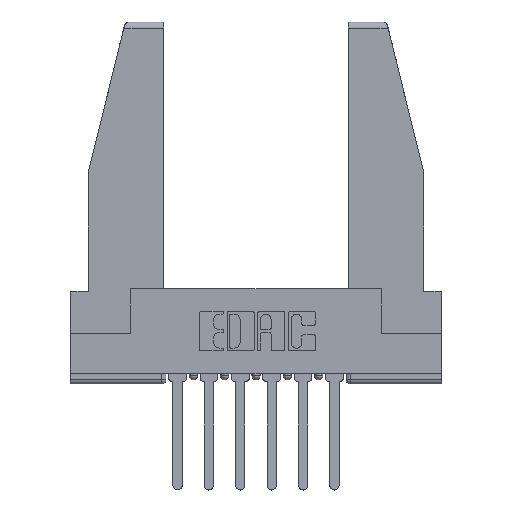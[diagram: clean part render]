
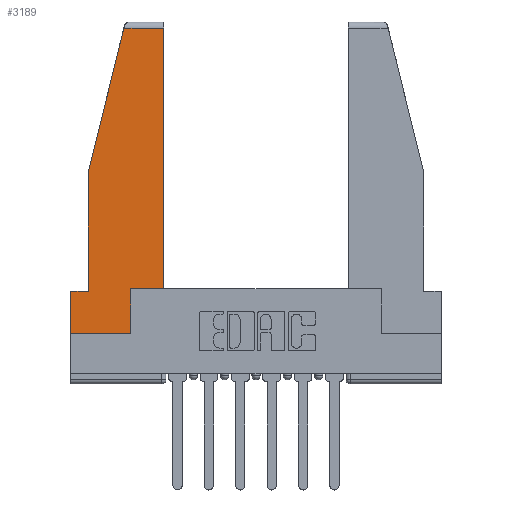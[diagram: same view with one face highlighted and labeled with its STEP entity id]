
A CAD part, top view. The second image highlights one B-rep face of the part: STEP entity #3189.
In plain terms, the highlighted planar face has unit normal (0, 0, 1).
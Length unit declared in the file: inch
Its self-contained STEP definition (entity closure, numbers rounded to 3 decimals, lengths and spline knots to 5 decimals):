
#70 = VERTEX_POINT ( 'NONE', #4856 ) ;
#126 = ORIENTED_EDGE ( 'NONE', *, *, #10428, .T. ) ;
#767 = VERTEX_POINT ( 'NONE', #4243 ) ;
#822 = EDGE_CURVE ( 'NONE', #12148, #7569, #9503, .T. ) ;
#844 = ORIENTED_EDGE ( 'NONE', *, *, #822, .T. ) ;
#858 = CARTESIAN_POINT ( 'NONE',  ( 0.086, 0.8, 0. ) ) ;
#1136 = PLANE ( 'NONE',  #5788 ) ;
#1160 = CARTESIAN_POINT ( 'NONE',  ( 0., 0., 0. ) ) ;
#1608 = CARTESIAN_POINT ( 'NONE',  ( 0., 0.21, 0. ) ) ;
#1762 = DIRECTION ( 'NONE',  ( 0., 1., 0. ) ) ;
#2064 = ORIENTED_EDGE ( 'NONE', *, *, #4403, .T. ) ;
#2156 = CARTESIAN_POINT ( 'NONE',  ( 0.271, 1.55, 0. ) ) ;
#2449 = DIRECTION ( 'NONE',  ( 1., 0., 0. ) ) ;
#3082 = DIRECTION ( 'NONE',  ( -0.239, -0.971, 0. ) ) ;
#3189 = ADVANCED_FACE ( 'NONE', ( #3199 ), #1136, .T. ) ;
#3199 = FACE_OUTER_BOUND ( 'NONE', #6763, .T. ) ;
#3532 = VECTOR ( 'NONE', #5253, 39.37008 ) ;
#3909 = EDGE_CURVE ( 'NONE', #70, #11465, #10698, .T. ) ;
#3946 = VECTOR ( 'NONE', #10074, 39.37008 ) ;
#4074 = EDGE_CURVE ( 'NONE', #6511, #70, #4246, .T. ) ;
#4205 = ORIENTED_EDGE ( 'NONE', *, *, #6234, .T. ) ;
#4243 = CARTESIAN_POINT ( 'NONE',  ( 0.297, 0., 0. ) ) ;
#4246 = LINE ( 'NONE', #8084, #3946 ) ;
#4403 = EDGE_CURVE ( 'NONE', #767, #12148, #9947, .T. ) ;
#4578 = CARTESIAN_POINT ( 'NONE',  ( 0.086, 0.21, 0. ) ) ;
#4725 = VECTOR ( 'NONE', #6793, 39.37008 ) ;
#4856 = CARTESIAN_POINT ( 'NONE',  ( 0.2636, 1.52, 0. ) ) ;
#5094 = CARTESIAN_POINT ( 'NONE',  ( 0., 0.21, 0. ) ) ;
#5253 = DIRECTION ( 'NONE',  ( 0., -1., 0. ) ) ;
#5254 = ORIENTED_EDGE ( 'NONE', *, *, #4074, .T. ) ;
#5375 = VECTOR ( 'NONE', #10734, 39.37008 ) ;
#5491 = CARTESIAN_POINT ( 'NONE',  ( 0.461, 0.223, 0. ) ) ;
#5518 = ORIENTED_EDGE ( 'NONE', *, *, #3909, .T. ) ;
#5684 = CARTESIAN_POINT ( 'NONE',  ( 0., 0.21, 0. ) ) ;
#5788 = AXIS2_PLACEMENT_3D ( 'NONE', #10563, #8725, #6898 ) ;
#5838 = VERTEX_POINT ( 'NONE', #8329 ) ;
#6207 = DIRECTION ( 'NONE',  ( 0., -1., 0. ) ) ;
#6234 = EDGE_CURVE ( 'NONE', #11465, #10917, #9386, .T. ) ;
#6461 = LINE ( 'NONE', #5094, #3532 ) ;
#6511 = VERTEX_POINT ( 'NONE', #9478 ) ;
#6543 = ORIENTED_EDGE ( 'NONE', *, *, #8089, .T. ) ;
#6763 = EDGE_LOOP ( 'NONE', ( #11177, #5254, #5518, #4205, #6543, #126, #9955, #2064, #844 ) ) ;
#6793 = DIRECTION ( 'NONE',  ( 1., 0., 0. ) ) ;
#6805 = LINE ( 'NONE', #5491, #7955 ) ;
#6880 = VECTOR ( 'NONE', #6207, 39.37008 ) ;
#6898 = DIRECTION ( 'NONE',  ( 1., 0., 0. ) ) ;
#6947 = CARTESIAN_POINT ( 'NONE',  ( 0.297, 0., 0. ) ) ;
#7335 = DIRECTION ( 'NONE',  ( -1., 0., 0. ) ) ;
#7569 = VERTEX_POINT ( 'NONE', #10974 ) ;
#7955 = VECTOR ( 'NONE', #1762, 39.37008 ) ;
#8084 = CARTESIAN_POINT ( 'NONE',  ( 0., 1.52, 0. ) ) ;
#8089 = EDGE_CURVE ( 'NONE', #10917, #9520, #11948, .T. ) ;
#8254 = VECTOR ( 'NONE', #7335, 39.37008 ) ;
#8329 = CARTESIAN_POINT ( 'NONE',  ( 0., 0., 0. ) ) ;
#8347 = CARTESIAN_POINT ( 'NONE',  ( 0.297, 0.223, 0. ) ) ;
#8725 = DIRECTION ( 'NONE',  ( 0., 0., 1. ) ) ;
#8764 = EDGE_CURVE ( 'NONE', #7569, #6511, #6805, .T. ) ;
#8935 = CARTESIAN_POINT ( 'NONE',  ( 0.086, 0.8, 0. ) ) ;
#9374 = VECTOR ( 'NONE', #3082, 39.37008 ) ;
#9386 = LINE ( 'NONE', #8935, #6880 ) ;
#9478 = CARTESIAN_POINT ( 'NONE',  ( 0.461, 1.52, 0. ) ) ;
#9503 = LINE ( 'NONE', #10431, #10085 ) ;
#9520 = VERTEX_POINT ( 'NONE', #5684 ) ;
#9707 = LINE ( 'NONE', #1160, #4725 ) ;
#9947 = LINE ( 'NONE', #6947, #5375 ) ;
#9955 = ORIENTED_EDGE ( 'NONE', *, *, #10263, .T. ) ;
#10074 = DIRECTION ( 'NONE',  ( -1., 0., 0. ) ) ;
#10085 = VECTOR ( 'NONE', #2449, 39.37008 ) ;
#10263 = EDGE_CURVE ( 'NONE', #5838, #767, #9707, .T. ) ;
#10428 = EDGE_CURVE ( 'NONE', #9520, #5838, #6461, .T. ) ;
#10431 = CARTESIAN_POINT ( 'NONE',  ( 0.297, 0.223, 0. ) ) ;
#10563 = CARTESIAN_POINT ( 'NONE',  ( 0., 0., 0. ) ) ;
#10698 = LINE ( 'NONE', #2156, #9374 ) ;
#10734 = DIRECTION ( 'NONE',  ( 0., 1., 0. ) ) ;
#10917 = VERTEX_POINT ( 'NONE', #4578 ) ;
#10974 = CARTESIAN_POINT ( 'NONE',  ( 0.461, 0.223, 0. ) ) ;
#11177 = ORIENTED_EDGE ( 'NONE', *, *, #8764, .T. ) ;
#11465 = VERTEX_POINT ( 'NONE', #858 ) ;
#11948 = LINE ( 'NONE', #1608, #8254 ) ;
#12148 = VERTEX_POINT ( 'NONE', #8347 ) ;
